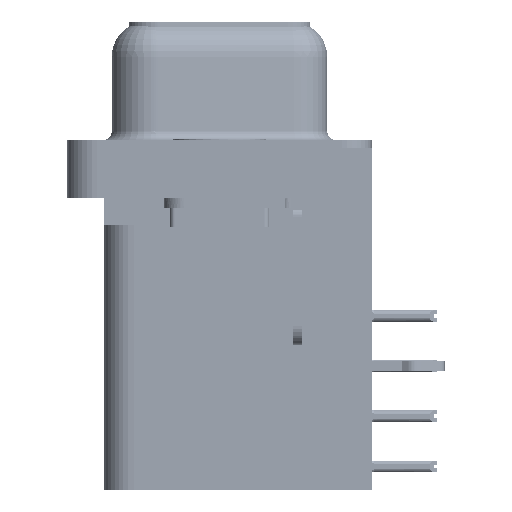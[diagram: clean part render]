
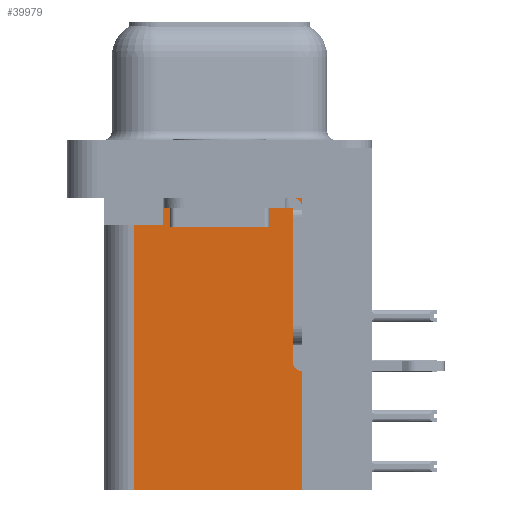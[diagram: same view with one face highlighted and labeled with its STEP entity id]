
A CAD part, left-side view. The second image highlights one B-rep face of the part: STEP entity #39979.
In plain terms, the highlighted planar face has unit normal (-1, 0, 0).
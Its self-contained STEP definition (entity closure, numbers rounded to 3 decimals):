
#155 = EDGE_LOOP ( 'NONE', ( #48722, #52251, #64728, #16275, #31503, #37405 ) ) ;
#1101 = CARTESIAN_POINT ( 'NONE',  ( 3.75, 0., -3.9 ) ) ;
#4931 = VERTEX_POINT ( 'NONE', #11368 ) ;
#5275 = VECTOR ( 'NONE', #43237, 1000. ) ;
#6050 = CARTESIAN_POINT ( 'NONE',  ( 3.75, -4.2, -17.3 ) ) ;
#6590 = VERTEX_POINT ( 'NONE', #39853 ) ;
#9916 = VERTEX_POINT ( 'NONE', #26988 ) ;
#10282 = LINE ( 'NONE', #57960, #49416 ) ;
#10431 = DIRECTION ( 'NONE',  ( 0., 1., 0. ) ) ;
#11368 = CARTESIAN_POINT ( 'NONE',  ( 3.75, 2.85, -3.9 ) ) ;
#11794 = DIRECTION ( 'NONE',  ( 1., 0., 0. ) ) ;
#16275 = ORIENTED_EDGE ( 'NONE', *, *, #67619, .F. ) ;
#16895 = PLANE ( 'NONE',  #61500 ) ;
#18821 = LINE ( 'NONE', #21508, #59734 ) ;
#21508 = CARTESIAN_POINT ( 'NONE',  ( 3.75, 2.85, -3.9 ) ) ;
#24664 = LINE ( 'NONE', #1101, #29648 ) ;
#25872 = EDGE_CURVE ( 'NONE', #9916, #4931, #18821, .T. ) ;
#26903 = DIRECTION ( 'NONE',  ( 0., 0., -1. ) ) ;
#26988 = CARTESIAN_POINT ( 'NONE',  ( 3.75, 2.85, -2.5 ) ) ;
#27283 = VECTOR ( 'NONE', #37398, 1000. ) ;
#28603 = CARTESIAN_POINT ( 'NONE',  ( 3.75, -4.2, -17.3 ) ) ;
#28926 = LINE ( 'NONE', #31811, #27283 ) ;
#29648 = VECTOR ( 'NONE', #38322, 1000. ) ;
#30207 = EDGE_CURVE ( 'NONE', #6590, #9916, #28926, .T. ) ;
#31503 = ORIENTED_EDGE ( 'NONE', *, *, #55824, .F. ) ;
#31811 = CARTESIAN_POINT ( 'NONE',  ( 3.75, -4.2, -2.5 ) ) ;
#37398 = DIRECTION ( 'NONE',  ( 0., 1., 0. ) ) ;
#37405 = ORIENTED_EDGE ( 'NONE', *, *, #60910, .T. ) ;
#38322 = DIRECTION ( 'NONE',  ( 0., 1., 0. ) ) ;
#39853 = CARTESIAN_POINT ( 'NONE',  ( 3.75, -4.2, -2.5 ) ) ;
#39979 = ADVANCED_FACE ( 'NONE', ( #52398 ), #16895, .F. ) ;
#41270 = EDGE_CURVE ( 'NONE', #4931, #63016, #24664, .T. ) ;
#43237 = DIRECTION ( 'NONE',  ( 0., 0., 1. ) ) ;
#45344 = LINE ( 'NONE', #50339, #59571 ) ;
#48722 = ORIENTED_EDGE ( 'NONE', *, *, #30207, .T. ) ;
#49043 = DIRECTION ( 'NONE',  ( 0., 1., 0. ) ) ;
#49416 = VECTOR ( 'NONE', #10431, 1000. ) ;
#50339 = CARTESIAN_POINT ( 'NONE',  ( 3.75, 4.35, -17.3 ) ) ;
#50519 = VERTEX_POINT ( 'NONE', #28603 ) ;
#50560 = DIRECTION ( 'NONE',  ( 0., 0., 1. ) ) ;
#52251 = ORIENTED_EDGE ( 'NONE', *, *, #25872, .T. ) ;
#52398 = FACE_OUTER_BOUND ( 'NONE', #155, .T. ) ;
#54668 = VERTEX_POINT ( 'NONE', #65870 ) ;
#55824 = EDGE_CURVE ( 'NONE', #50519, #54668, #10282, .T. ) ;
#57960 = CARTESIAN_POINT ( 'NONE',  ( 3.75, -4.2, -17.3 ) ) ;
#59571 = VECTOR ( 'NONE', #50560, 1000. ) ;
#59734 = VECTOR ( 'NONE', #26903, 1000. ) ;
#60264 = LINE ( 'NONE', #6050, #5275 ) ;
#60910 = EDGE_CURVE ( 'NONE', #50519, #6590, #60264, .T. ) ;
#61500 = AXIS2_PLACEMENT_3D ( 'NONE', #64940, #11794, #49043 ) ;
#63016 = VERTEX_POINT ( 'NONE', #63043 ) ;
#63043 = CARTESIAN_POINT ( 'NONE',  ( 3.75, 4.35, -3.9 ) ) ;
#64728 = ORIENTED_EDGE ( 'NONE', *, *, #41270, .T. ) ;
#64940 = CARTESIAN_POINT ( 'NONE',  ( 3.75, -4.2, -17.3 ) ) ;
#65870 = CARTESIAN_POINT ( 'NONE',  ( 3.75, 4.35, -17.3 ) ) ;
#67619 = EDGE_CURVE ( 'NONE', #54668, #63016, #45344, .T. ) ;
